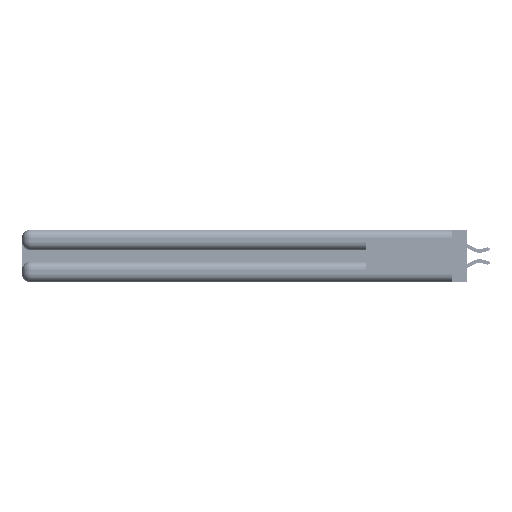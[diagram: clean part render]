
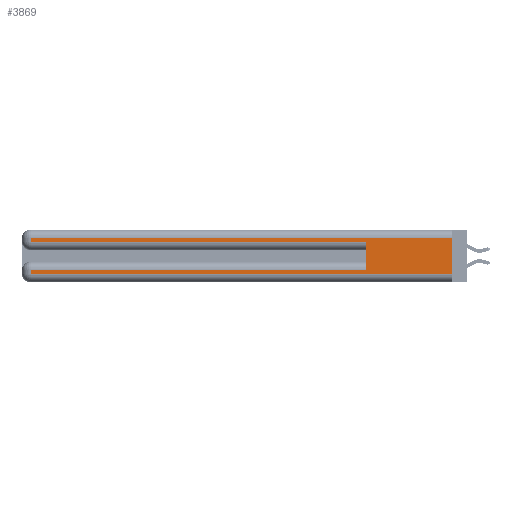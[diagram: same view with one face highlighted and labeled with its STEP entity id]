
A CAD part, left-side view. The second image highlights one B-rep face of the part: STEP entity #3869.
In plain terms, the highlighted planar face has unit normal (-1, 0, 0).
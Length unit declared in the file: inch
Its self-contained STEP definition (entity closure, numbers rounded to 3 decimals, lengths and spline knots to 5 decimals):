
#4 = VECTOR ( 'NONE', #22473, 39.37008 ) ;
#200 = CARTESIAN_POINT ( 'NONE',  ( 0., 2.94, 0.37 ) ) ;
#486 = CARTESIAN_POINT ( 'NONE',  ( 0., 0., 0.31 ) ) ;
#1615 = LINE ( 'NONE', #39616, #2283 ) ;
#1859 = DIRECTION ( 'NONE',  ( 0., 1., 0. ) ) ;
#2135 = LINE ( 'NONE', #30207, #18763 ) ;
#2180 = ORIENTED_EDGE ( 'NONE', *, *, #51782, .F. ) ;
#2283 = VECTOR ( 'NONE', #8300, 39.37008 ) ;
#3575 = DIRECTION ( 'NONE',  ( 0., 0., -1. ) ) ;
#3869 = ADVANCED_FACE ( 'NONE', ( #21418 ), #38193, .F. ) ;
#4285 = ORIENTED_EDGE ( 'NONE', *, *, #13015, .F. ) ;
#4380 = VERTEX_POINT ( 'NONE', #19587 ) ;
#4622 = VERTEX_POINT ( 'NONE', #22058 ) ;
#5755 = VERTEX_POINT ( 'NONE', #40323 ) ;
#8300 = DIRECTION ( 'NONE',  ( 0., 0., 1. ) ) ;
#8393 = EDGE_CURVE ( 'NONE', #4622, #4380, #30717, .T. ) ;
#8423 = CARTESIAN_POINT ( 'NONE',  ( 0., 0., 0.37 ) ) ;
#10850 = DIRECTION ( 'NONE',  ( 0., 0., -1. ) ) ;
#12770 = DIRECTION ( 'NONE',  ( 0., 0., -1. ) ) ;
#13015 = EDGE_CURVE ( 'NONE', #5755, #23818, #1615, .T. ) ;
#13460 = LINE ( 'NONE', #15072, #47360 ) ;
#13527 = LINE ( 'NONE', #41739, #16307 ) ;
#15072 = CARTESIAN_POINT ( 'NONE',  ( 0., 0., 0.31 ) ) ;
#15267 = DIRECTION ( 'NONE',  ( 0., -1., 0. ) ) ;
#15513 = ORIENTED_EDGE ( 'NONE', *, *, #22632, .T. ) ;
#16307 = VECTOR ( 'NONE', #15267, 39.37008 ) ;
#17057 = VECTOR ( 'NONE', #44533, 39.37008 ) ;
#17548 = VECTOR ( 'NONE', #10850, 39.37008 ) ;
#18763 = VECTOR ( 'NONE', #12770, 39.37008 ) ;
#19021 = EDGE_CURVE ( 'NONE', #5755, #31373, #35471, .T. ) ;
#19587 = CARTESIAN_POINT ( 'NONE',  ( 0., 2.94, 0.285 ) ) ;
#19889 = DIRECTION ( 'NONE',  ( 0., 1., 0. ) ) ;
#21319 = ORIENTED_EDGE ( 'NONE', *, *, #55875, .T. ) ;
#21418 = FACE_OUTER_BOUND ( 'NONE', #33032, .T. ) ;
#22058 = CARTESIAN_POINT ( 'NONE',  ( 0., 2.94, 0.31 ) ) ;
#22473 = DIRECTION ( 'NONE',  ( 0., -1., 0. ) ) ;
#22632 = EDGE_CURVE ( 'NONE', #31373, #46531, #29543, .T. ) ;
#23686 = ORIENTED_EDGE ( 'NONE', *, *, #19021, .T. ) ;
#23818 = VERTEX_POINT ( 'NONE', #30693 ) ;
#26108 = EDGE_CURVE ( 'NONE', #4380, #23818, #36729, .T. ) ;
#29543 = LINE ( 'NONE', #200, #17057 ) ;
#30207 = CARTESIAN_POINT ( 'NONE',  ( 0., 0., 0.37 ) ) ;
#30693 = CARTESIAN_POINT ( 'NONE',  ( 0., 0.6, 0.285 ) ) ;
#30717 = LINE ( 'NONE', #32915, #17548 ) ;
#31373 = VERTEX_POINT ( 'NONE', #49272 ) ;
#32915 = CARTESIAN_POINT ( 'NONE',  ( 0., 2.94, 0.37 ) ) ;
#33032 = EDGE_LOOP ( 'NONE', ( #2180, #43062, #36800, #41808, #4285, #23686, #15513, #21319 ) ) ;
#34917 = DIRECTION ( 'NONE',  ( 1., 0., 0. ) ) ;
#35213 = AXIS2_PLACEMENT_3D ( 'NONE', #8423, #34917, #3575 ) ;
#35471 = LINE ( 'NONE', #41562, #54852 ) ;
#36729 = LINE ( 'NONE', #53283, #4 ) ;
#36800 = ORIENTED_EDGE ( 'NONE', *, *, #8393, .T. ) ;
#37357 = VERTEX_POINT ( 'NONE', #486 ) ;
#38193 = PLANE ( 'NONE',  #35213 ) ;
#39616 = CARTESIAN_POINT ( 'NONE',  ( 0., 0.6, 0.145 ) ) ;
#40323 = CARTESIAN_POINT ( 'NONE',  ( 0., 0.6, 0.085 ) ) ;
#41562 = CARTESIAN_POINT ( 'NONE',  ( 0., 0., 0.085 ) ) ;
#41739 = CARTESIAN_POINT ( 'NONE',  ( 0., 0., 0.06 ) ) ;
#41808 = ORIENTED_EDGE ( 'NONE', *, *, #26108, .T. ) ;
#43062 = ORIENTED_EDGE ( 'NONE', *, *, #50457, .T. ) ;
#44533 = DIRECTION ( 'NONE',  ( 0., 0., -1. ) ) ;
#44633 = VERTEX_POINT ( 'NONE', #47024 ) ;
#46531 = VERTEX_POINT ( 'NONE', #52059 ) ;
#47024 = CARTESIAN_POINT ( 'NONE',  ( 0., 0., 0.06 ) ) ;
#47360 = VECTOR ( 'NONE', #1859, 39.37008 ) ;
#49272 = CARTESIAN_POINT ( 'NONE',  ( 0., 2.94, 0.085 ) ) ;
#50457 = EDGE_CURVE ( 'NONE', #37357, #4622, #13460, .T. ) ;
#51782 = EDGE_CURVE ( 'NONE', #37357, #44633, #2135, .T. ) ;
#52059 = CARTESIAN_POINT ( 'NONE',  ( 0., 2.94, 0.06 ) ) ;
#53283 = CARTESIAN_POINT ( 'NONE',  ( 0., 0., 0.285 ) ) ;
#54852 = VECTOR ( 'NONE', #19889, 39.37008 ) ;
#55875 = EDGE_CURVE ( 'NONE', #46531, #44633, #13527, .T. ) ;
